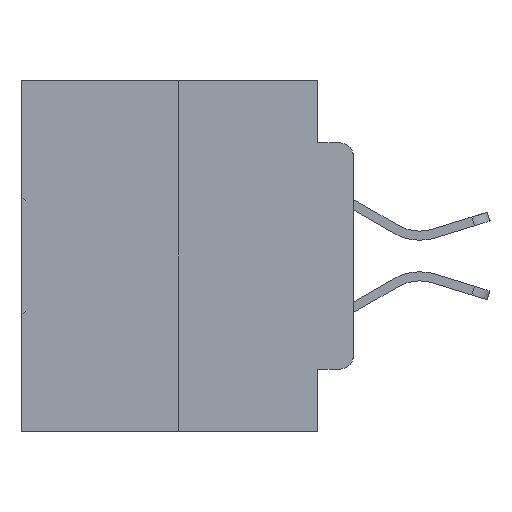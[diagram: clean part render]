
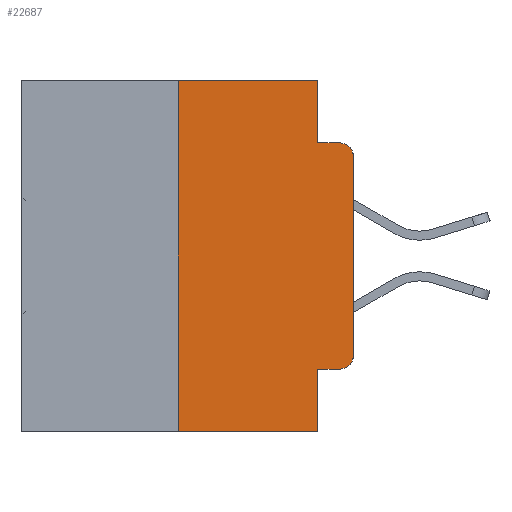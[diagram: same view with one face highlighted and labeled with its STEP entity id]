
A CAD part, left-side view. The second image highlights one B-rep face of the part: STEP entity #22687.
In plain terms, the highlighted planar face has unit normal (-1, 0, 0).
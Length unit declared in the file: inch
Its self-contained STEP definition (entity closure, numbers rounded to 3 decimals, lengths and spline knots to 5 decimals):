
#43 = EDGE_LOOP ( 'NONE', ( #10493, #30563, #12051, #14341, #27204, #2712, #28708, #29467, #17427, #24581 ) ) ;
#57 = VECTOR ( 'NONE', #19620, 39.37008 ) ;
#1144 = LINE ( 'NONE', #2591, #13576 ) ;
#1422 = DIRECTION ( 'NONE',  ( 0., -1., 0. ) ) ;
#2304 = CARTESIAN_POINT ( 'NONE',  ( 0., 0.051, -0.0885 ) ) ;
#2327 = VERTEX_POINT ( 'NONE', #9175 ) ;
#2591 = CARTESIAN_POINT ( 'NONE',  ( 0., 0.051, 0. ) ) ;
#2696 = DIRECTION ( 'NONE',  ( 0., 0., -1. ) ) ;
#2704 = VERTEX_POINT ( 'NONE', #19932 ) ;
#2712 = ORIENTED_EDGE ( 'NONE', *, *, #10636, .F. ) ;
#3045 = CARTESIAN_POINT ( 'NONE',  ( 0., 0.25, -0.5 ) ) ;
#3499 = LINE ( 'NONE', #6413, #15875 ) ;
#3774 = CARTESIAN_POINT ( 'NONE',  ( 0., 0., -0.1085 ) ) ;
#4071 = EDGE_CURVE ( 'NONE', #13026, #2704, #21189, .T. ) ;
#5195 = CARTESIAN_POINT ( 'NONE',  ( 0., 0., 0. ) ) ;
#5450 = LINE ( 'NONE', #21083, #30549 ) ;
#6413 = CARTESIAN_POINT ( 'NONE',  ( 0., 0.473, -0.5 ) ) ;
#6647 = LINE ( 'NONE', #19879, #12467 ) ;
#7011 = VERTEX_POINT ( 'NONE', #3774 ) ;
#7097 = VECTOR ( 'NONE', #22646, 39.37008 ) ;
#7736 = DIRECTION ( 'NONE',  ( -1., 0., 0. ) ) ;
#7937 = VERTEX_POINT ( 'NONE', #3045 ) ;
#8896 = DIRECTION ( 'NONE',  ( 0., -1., 0. ) ) ;
#9175 = CARTESIAN_POINT ( 'NONE',  ( 0., 0.051, 0. ) ) ;
#9784 = DIRECTION ( 'NONE',  ( 1., 0., 0. ) ) ;
#10452 = EDGE_CURVE ( 'NONE', #27740, #18630, #19092, .T. ) ;
#10493 = ORIENTED_EDGE ( 'NONE', *, *, #29479, .T. ) ;
#10636 = EDGE_CURVE ( 'NONE', #7937, #26502, #20212, .T. ) ;
#12051 = ORIENTED_EDGE ( 'NONE', *, *, #10452, .F. ) ;
#12467 = VECTOR ( 'NONE', #2696, 39.37008 ) ;
#12470 = EDGE_CURVE ( 'NONE', #19604, #13288, #6647, .T. ) ;
#12478 = AXIS2_PLACEMENT_3D ( 'NONE', #22451, #7736, #24838 ) ;
#12522 = VECTOR ( 'NONE', #26269, 39.37008 ) ;
#13026 = VERTEX_POINT ( 'NONE', #17272 ) ;
#13288 = VERTEX_POINT ( 'NONE', #20640 ) ;
#13383 = LINE ( 'NONE', #5195, #25527 ) ;
#13576 = VECTOR ( 'NONE', #17418, 39.37008 ) ;
#14341 = ORIENTED_EDGE ( 'NONE', *, *, #25569, .F. ) ;
#15875 = VECTOR ( 'NONE', #8896, 39.37008 ) ;
#16573 = CARTESIAN_POINT ( 'NONE',  ( 0., 0.051, -0.4115 ) ) ;
#17095 = CARTESIAN_POINT ( 'NONE',  ( 0., 0.473, 0. ) ) ;
#17272 = CARTESIAN_POINT ( 'NONE',  ( 0., 0.02, -0.4115 ) ) ;
#17418 = DIRECTION ( 'NONE',  ( 0., 0., -1. ) ) ;
#17427 = ORIENTED_EDGE ( 'NONE', *, *, #19359, .T. ) ;
#17519 = LINE ( 'NONE', #16573, #12522 ) ;
#17780 = CARTESIAN_POINT ( 'NONE',  ( 0., 0.25, 0. ) ) ;
#18630 = VERTEX_POINT ( 'NONE', #28390 ) ;
#19092 = LINE ( 'NONE', #2304, #57 ) ;
#19309 = DIRECTION ( 'NONE',  ( -1., 0., 0. ) ) ;
#19359 = EDGE_CURVE ( 'NONE', #19604, #13026, #17519, .T. ) ;
#19372 = CARTESIAN_POINT ( 'NONE',  ( 0., 0.02, -0.3915 ) ) ;
#19604 = VERTEX_POINT ( 'NONE', #22392 ) ;
#19620 = DIRECTION ( 'NONE',  ( 0., -1., 0. ) ) ;
#19879 = CARTESIAN_POINT ( 'NONE',  ( 0., 0.051, 0. ) ) ;
#19932 = CARTESIAN_POINT ( 'NONE',  ( 0., 0., -0.3915 ) ) ;
#20212 = LINE ( 'NONE', #17780, #7097 ) ;
#20640 = CARTESIAN_POINT ( 'NONE',  ( 0., 0.051, -0.5 ) ) ;
#20663 = EDGE_CURVE ( 'NONE', #7937, #13288, #3499, .T. ) ;
#20741 = CARTESIAN_POINT ( 'NONE',  ( 0., 0.051, -0.0885 ) ) ;
#21083 = CARTESIAN_POINT ( 'NONE',  ( 0., 0.473, 0. ) ) ;
#21189 = CIRCLE ( 'NONE', #30013, 0.02 ) ;
#22392 = CARTESIAN_POINT ( 'NONE',  ( 0., 0.051, -0.4115 ) ) ;
#22451 = CARTESIAN_POINT ( 'NONE',  ( 0., 0.02, -0.1085 ) ) ;
#22553 = FACE_OUTER_BOUND ( 'NONE', #43, .T. ) ;
#22646 = DIRECTION ( 'NONE',  ( 0., 0., 1. ) ) ;
#22687 = ADVANCED_FACE ( 'NONE', ( #22553 ), #24356, .F. ) ;
#24356 = PLANE ( 'NONE',  #29801 ) ;
#24581 = ORIENTED_EDGE ( 'NONE', *, *, #4071, .T. ) ;
#24722 = DIRECTION ( 'NONE',  ( 0., 0., -1. ) ) ;
#24838 = DIRECTION ( 'NONE',  ( 0., 0., -1. ) ) ;
#24993 = CARTESIAN_POINT ( 'NONE',  ( 0., 0.25, 0. ) ) ;
#25527 = VECTOR ( 'NONE', #29556, 39.37008 ) ;
#25569 = EDGE_CURVE ( 'NONE', #2327, #27740, #1144, .T. ) ;
#26269 = DIRECTION ( 'NONE',  ( 0., -1., 0. ) ) ;
#26502 = VERTEX_POINT ( 'NONE', #24993 ) ;
#26786 = DIRECTION ( 'NONE',  ( 0., 0., -1. ) ) ;
#27204 = ORIENTED_EDGE ( 'NONE', *, *, #27316, .F. ) ;
#27316 = EDGE_CURVE ( 'NONE', #26502, #2327, #5450, .T. ) ;
#27740 = VERTEX_POINT ( 'NONE', #20741 ) ;
#28390 = CARTESIAN_POINT ( 'NONE',  ( 0., 0.02, -0.0885 ) ) ;
#28708 = ORIENTED_EDGE ( 'NONE', *, *, #20663, .T. ) ;
#29467 = ORIENTED_EDGE ( 'NONE', *, *, #12470, .F. ) ;
#29479 = EDGE_CURVE ( 'NONE', #2704, #7011, #13383, .T. ) ;
#29541 = CIRCLE ( 'NONE', #12478, 0.02 ) ;
#29556 = DIRECTION ( 'NONE',  ( 0., 0., 1. ) ) ;
#29801 = AXIS2_PLACEMENT_3D ( 'NONE', #17095, #9784, #26786 ) ;
#30013 = AXIS2_PLACEMENT_3D ( 'NONE', #19372, #19309, #24722 ) ;
#30549 = VECTOR ( 'NONE', #1422, 39.37008 ) ;
#30563 = ORIENTED_EDGE ( 'NONE', *, *, #31312, .T. ) ;
#31312 = EDGE_CURVE ( 'NONE', #7011, #18630, #29541, .T. ) ;
